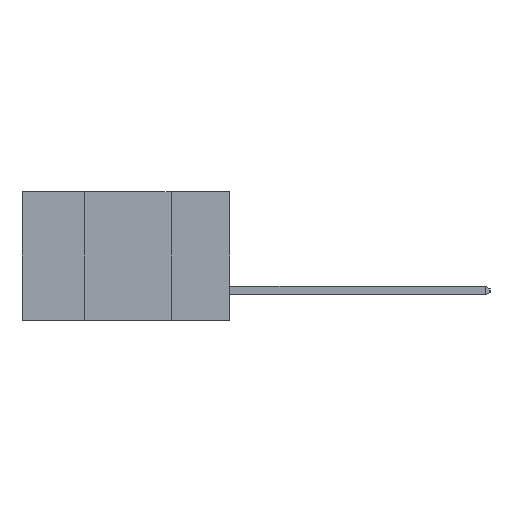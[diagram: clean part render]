
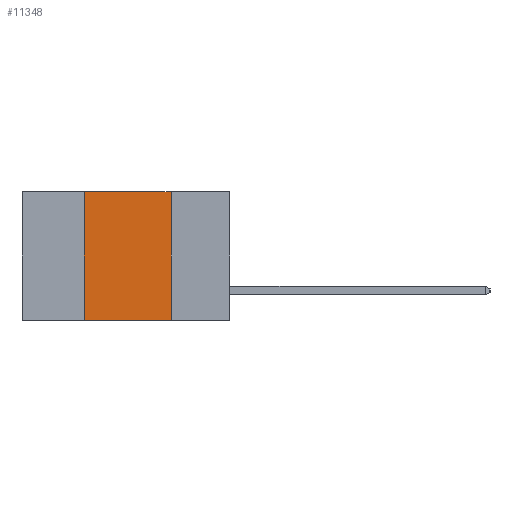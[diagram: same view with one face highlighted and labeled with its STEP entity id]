
A CAD part, left-side view. The second image highlights one B-rep face of the part: STEP entity #11348.
In plain terms, the highlighted planar face has unit normal (-1, 0, 0).
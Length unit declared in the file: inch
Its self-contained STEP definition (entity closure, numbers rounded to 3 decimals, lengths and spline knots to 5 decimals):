
#842 = VECTOR ( 'NONE', #10455, 39.37008 ) ;
#1336 = LINE ( 'NONE', #5768, #842 ) ;
#1551 = DIRECTION ( 'NONE',  ( 0., -1., 0. ) ) ;
#1592 = PLANE ( 'NONE',  #3531 ) ;
#1998 = EDGE_LOOP ( 'NONE', ( #19804, #4329, #16673, #13064 ) ) ;
#2848 = LINE ( 'NONE', #8248, #14290 ) ;
#3531 = AXIS2_PLACEMENT_3D ( 'NONE', #15549, #18657, #9403 ) ;
#3541 = VERTEX_POINT ( 'NONE', #16438 ) ;
#4151 = CARTESIAN_POINT ( 'NONE',  ( 0., 0.42, 0. ) ) ;
#4329 = ORIENTED_EDGE ( 'NONE', *, *, #13206, .F. ) ;
#5211 = CARTESIAN_POINT ( 'NONE',  ( 0., 0.42, -0.37 ) ) ;
#5768 = CARTESIAN_POINT ( 'NONE',  ( 0., 0.17, 0. ) ) ;
#6293 = CARTESIAN_POINT ( 'NONE',  ( 0., 0.6, 0. ) ) ;
#6748 = FACE_OUTER_BOUND ( 'NONE', #1998, .T. ) ;
#8248 = CARTESIAN_POINT ( 'NONE',  ( 0., 0.6, -0.37 ) ) ;
#8691 = VERTEX_POINT ( 'NONE', #4151 ) ;
#8846 = LINE ( 'NONE', #6293, #13982 ) ;
#9259 = CARTESIAN_POINT ( 'NONE',  ( 0., 0.42, 0. ) ) ;
#9403 = DIRECTION ( 'NONE',  ( 0., 0., -1. ) ) ;
#10455 = DIRECTION ( 'NONE',  ( 0., 0., -1. ) ) ;
#10871 = EDGE_CURVE ( 'NONE', #19280, #14374, #2848, .T. ) ;
#11348 = ADVANCED_FACE ( 'NONE', ( #6748 ), #1592, .F. ) ;
#11915 = EDGE_CURVE ( 'NONE', #19280, #8691, #17648, .T. ) ;
#12938 = EDGE_CURVE ( 'NONE', #3541, #14374, #1336, .T. ) ;
#13064 = ORIENTED_EDGE ( 'NONE', *, *, #10871, .T. ) ;
#13206 = EDGE_CURVE ( 'NONE', #8691, #3541, #8846, .T. ) ;
#13982 = VECTOR ( 'NONE', #1551, 39.37008 ) ;
#14290 = VECTOR ( 'NONE', #16038, 39.37008 ) ;
#14374 = VERTEX_POINT ( 'NONE', #19479 ) ;
#15549 = CARTESIAN_POINT ( 'NONE',  ( 0., 0.6, 0. ) ) ;
#16038 = DIRECTION ( 'NONE',  ( 0., -1., 0. ) ) ;
#16438 = CARTESIAN_POINT ( 'NONE',  ( 0., 0.17, 0. ) ) ;
#16665 = VECTOR ( 'NONE', #18525, 39.37008 ) ;
#16673 = ORIENTED_EDGE ( 'NONE', *, *, #11915, .F. ) ;
#17648 = LINE ( 'NONE', #9259, #16665 ) ;
#18525 = DIRECTION ( 'NONE',  ( 0., 0., 1. ) ) ;
#18657 = DIRECTION ( 'NONE',  ( 1., 0., 0. ) ) ;
#19280 = VERTEX_POINT ( 'NONE', #5211 ) ;
#19479 = CARTESIAN_POINT ( 'NONE',  ( 0., 0.17, -0.37 ) ) ;
#19804 = ORIENTED_EDGE ( 'NONE', *, *, #12938, .F. ) ;
